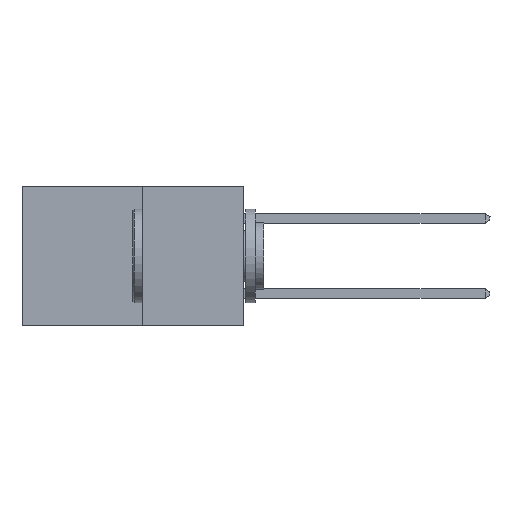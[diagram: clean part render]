
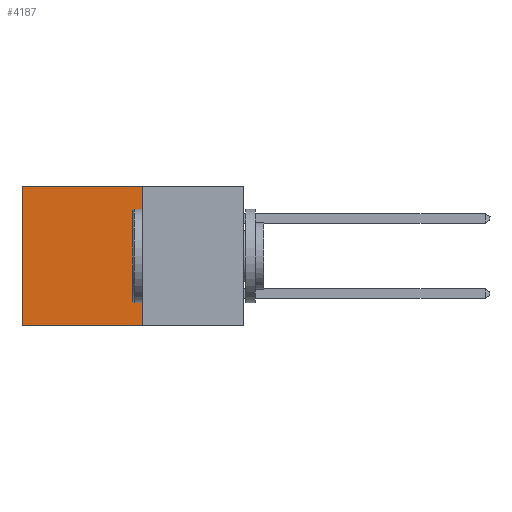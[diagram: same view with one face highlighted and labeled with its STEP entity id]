
A CAD part, left-side view. The second image highlights one B-rep face of the part: STEP entity #4187.
In plain terms, the highlighted planar face has unit normal (-1, 0, 0).
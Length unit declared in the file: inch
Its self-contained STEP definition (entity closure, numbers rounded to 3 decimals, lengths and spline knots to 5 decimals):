
#796 = CARTESIAN_POINT ( 'NONE',  ( 0.277, 0.59, -0.37 ) ) ;
#1616 = EDGE_CURVE ( 'NONE', #13687, #6621, #15002, .T. ) ;
#1949 = DIRECTION ( 'NONE',  ( 0., 1., 0. ) ) ;
#3866 = VERTEX_POINT ( 'NONE', #7852 ) ;
#4187 = ADVANCED_FACE ( 'NONE', ( #13976 ), #11286, .F. ) ;
#4204 = DIRECTION ( 'NONE',  ( 0., 0., -1. ) ) ;
#4294 = ORIENTED_EDGE ( 'NONE', *, *, #1616, .F. ) ;
#4373 = CARTESIAN_POINT ( 'NONE',  ( 0.277, 0.59, 0. ) ) ;
#4995 = DIRECTION ( 'NONE',  ( 0., 1., 0. ) ) ;
#5110 = CARTESIAN_POINT ( 'NONE',  ( 0.277, 0.27, 0. ) ) ;
#5200 = VECTOR ( 'NONE', #4995, 39.37008 ) ;
#6621 = VERTEX_POINT ( 'NONE', #8429 ) ;
#7139 = VERTEX_POINT ( 'NONE', #4373 ) ;
#7273 = ORIENTED_EDGE ( 'NONE', *, *, #11474, .T. ) ;
#7568 = EDGE_LOOP ( 'NONE', ( #7273, #4294, #8038, #11768 ) ) ;
#7852 = CARTESIAN_POINT ( 'NONE',  ( 0.277, 0.27, 0. ) ) ;
#8038 = ORIENTED_EDGE ( 'NONE', *, *, #13691, .F. ) ;
#8110 = DIRECTION ( 'NONE',  ( 0., 0., -1. ) ) ;
#8396 = VECTOR ( 'NONE', #1949, 39.37008 ) ;
#8429 = CARTESIAN_POINT ( 'NONE',  ( 0.277, 0.59, -0.37 ) ) ;
#8768 = EDGE_CURVE ( 'NONE', #3866, #7139, #15190, .T. ) ;
#9456 = CARTESIAN_POINT ( 'NONE',  ( 0.277, 0.27, -0.37 ) ) ;
#9705 = VECTOR ( 'NONE', #4204, 39.37008 ) ;
#10371 = DIRECTION ( 'NONE',  ( 0., 0., -1. ) ) ;
#10973 = DIRECTION ( 'NONE',  ( 1., 0., 0. ) ) ;
#11089 = CARTESIAN_POINT ( 'NONE',  ( 0.277, 0.27, -0.37 ) ) ;
#11286 = PLANE ( 'NONE',  #12884 ) ;
#11474 = EDGE_CURVE ( 'NONE', #7139, #6621, #13371, .T. ) ;
#11768 = ORIENTED_EDGE ( 'NONE', *, *, #8768, .T. ) ;
#12884 = AXIS2_PLACEMENT_3D ( 'NONE', #11089, #10973, #10371 ) ;
#12909 = VECTOR ( 'NONE', #8110, 39.37008 ) ;
#13283 = LINE ( 'NONE', #15552, #12909 ) ;
#13371 = LINE ( 'NONE', #796, #9705 ) ;
#13687 = VERTEX_POINT ( 'NONE', #14301 ) ;
#13691 = EDGE_CURVE ( 'NONE', #3866, #13687, #13283, .T. ) ;
#13976 = FACE_OUTER_BOUND ( 'NONE', #7568, .T. ) ;
#14301 = CARTESIAN_POINT ( 'NONE',  ( 0.277, 0.27, -0.37 ) ) ;
#15002 = LINE ( 'NONE', #9456, #8396 ) ;
#15190 = LINE ( 'NONE', #5110, #5200 ) ;
#15552 = CARTESIAN_POINT ( 'NONE',  ( 0.277, 0.27, -0.37 ) ) ;
